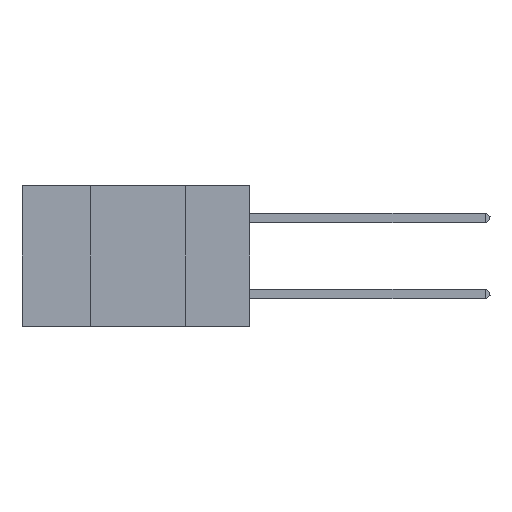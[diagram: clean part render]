
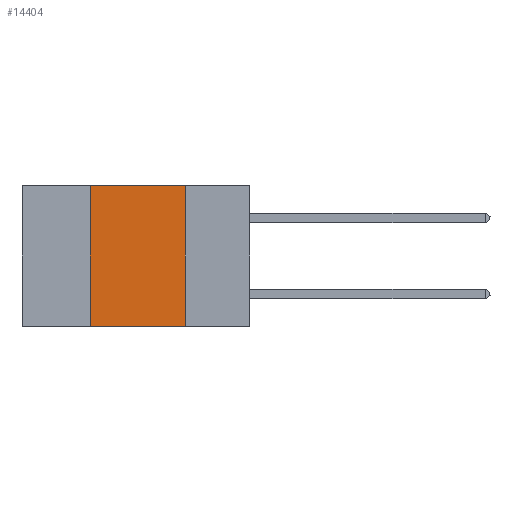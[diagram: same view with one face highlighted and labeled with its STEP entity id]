
A CAD part, left-side view. The second image highlights one B-rep face of the part: STEP entity #14404.
In plain terms, the highlighted planar face has unit normal (-1, 0, 0).
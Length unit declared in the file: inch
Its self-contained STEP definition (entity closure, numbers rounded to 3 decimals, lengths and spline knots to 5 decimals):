
#618 = ORIENTED_EDGE ( 'NONE', *, *, #27060, .F. ) ;
#852 = CARTESIAN_POINT ( 'NONE',  ( 0., 0.42, 0. ) ) ;
#1601 = CARTESIAN_POINT ( 'NONE',  ( 0., 0.6, -0.37 ) ) ;
#3267 = EDGE_CURVE ( 'NONE', #17010, #3685, #3651, .T. ) ;
#3651 = LINE ( 'NONE', #12668, #28406 ) ;
#3685 = VERTEX_POINT ( 'NONE', #852 ) ;
#4334 = ORIENTED_EDGE ( 'NONE', *, *, #3267, .F. ) ;
#4719 = VECTOR ( 'NONE', #28003, 39.37008 ) ;
#5251 = EDGE_CURVE ( 'NONE', #17010, #19591, #28319, .T. ) ;
#6061 = EDGE_CURVE ( 'NONE', #3685, #18198, #25300, .T. ) ;
#8209 = CARTESIAN_POINT ( 'NONE',  ( 0., 0.17, 0. ) ) ;
#8456 = VECTOR ( 'NONE', #22894, 39.37008 ) ;
#8607 = DIRECTION ( 'NONE',  ( 0., -1., 0. ) ) ;
#9092 = ORIENTED_EDGE ( 'NONE', *, *, #5251, .T. ) ;
#9724 = PLANE ( 'NONE',  #18717 ) ;
#11339 = CARTESIAN_POINT ( 'NONE',  ( 0., 0.17, 0. ) ) ;
#11996 = CARTESIAN_POINT ( 'NONE',  ( 0., 0.6, 0. ) ) ;
#12668 = CARTESIAN_POINT ( 'NONE',  ( 0., 0.42, 0. ) ) ;
#13337 = ORIENTED_EDGE ( 'NONE', *, *, #6061, .F. ) ;
#14404 = ADVANCED_FACE ( 'NONE', ( #28045 ), #9724, .F. ) ;
#16944 = DIRECTION ( 'NONE',  ( 1., 0., 0. ) ) ;
#17010 = VERTEX_POINT ( 'NONE', #18109 ) ;
#17584 = DIRECTION ( 'NONE',  ( 0., 0., 1. ) ) ;
#18109 = CARTESIAN_POINT ( 'NONE',  ( 0., 0.42, -0.37 ) ) ;
#18198 = VERTEX_POINT ( 'NONE', #8209 ) ;
#18614 = LINE ( 'NONE', #11339, #4719 ) ;
#18717 = AXIS2_PLACEMENT_3D ( 'NONE', #11996, #16944, #26066 ) ;
#19026 = EDGE_LOOP ( 'NONE', ( #618, #13337, #4334, #9092 ) ) ;
#19591 = VERTEX_POINT ( 'NONE', #21033 ) ;
#20576 = CARTESIAN_POINT ( 'NONE',  ( 0., 0.6, 0. ) ) ;
#21033 = CARTESIAN_POINT ( 'NONE',  ( 0., 0.17, -0.37 ) ) ;
#22894 = DIRECTION ( 'NONE',  ( 0., -1., 0. ) ) ;
#25300 = LINE ( 'NONE', #20576, #28293 ) ;
#26066 = DIRECTION ( 'NONE',  ( 0., 0., -1. ) ) ;
#27060 = EDGE_CURVE ( 'NONE', #18198, #19591, #18614, .T. ) ;
#28003 = DIRECTION ( 'NONE',  ( 0., 0., -1. ) ) ;
#28045 = FACE_OUTER_BOUND ( 'NONE', #19026, .T. ) ;
#28293 = VECTOR ( 'NONE', #8607, 39.37008 ) ;
#28319 = LINE ( 'NONE', #1601, #8456 ) ;
#28406 = VECTOR ( 'NONE', #17584, 39.37008 ) ;
